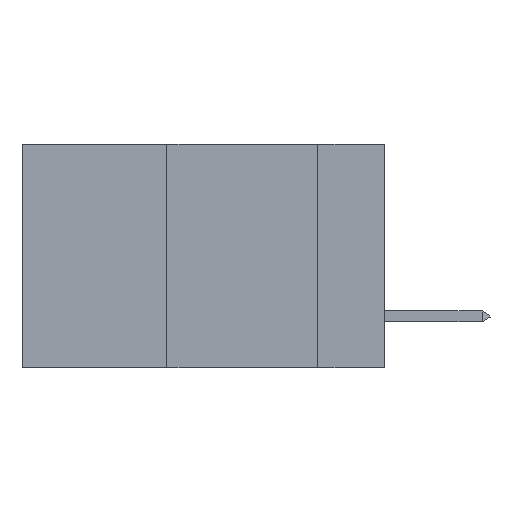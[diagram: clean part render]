
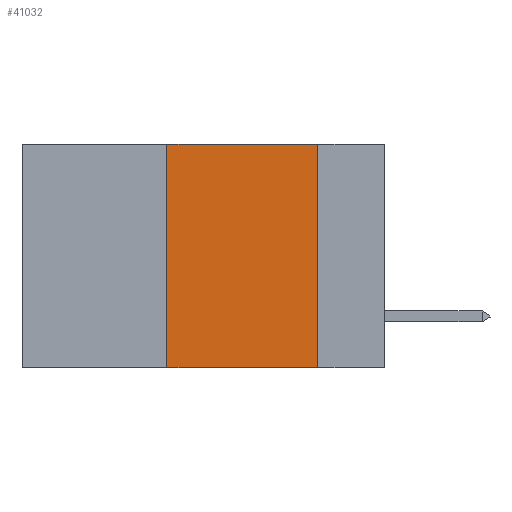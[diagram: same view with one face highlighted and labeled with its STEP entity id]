
A CAD part, left-side view. The second image highlights one B-rep face of the part: STEP entity #41032.
In plain terms, the highlighted planar face has unit normal (-1, 0, 0).
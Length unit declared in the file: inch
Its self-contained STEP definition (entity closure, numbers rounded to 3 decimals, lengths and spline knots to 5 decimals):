
#2736 = VERTEX_POINT ( 'NONE', #15024 ) ;
#3835 = CARTESIAN_POINT ( 'NONE',  ( 0., 0.11, 0. ) ) ;
#3850 = VECTOR ( 'NONE', #11219, 39.37008 ) ;
#7712 = EDGE_LOOP ( 'NONE', ( #29651, #24630, #30000, #11741 ) ) ;
#8691 = CARTESIAN_POINT ( 'NONE',  ( 0., 0.6, -0.37 ) ) ;
#10247 = CARTESIAN_POINT ( 'NONE',  ( 0., 0.36, -0.37 ) ) ;
#10599 = CARTESIAN_POINT ( 'NONE',  ( 0., 0.36, 0. ) ) ;
#11119 = CARTESIAN_POINT ( 'NONE',  ( 0., 0.36, 0. ) ) ;
#11219 = DIRECTION ( 'NONE',  ( 0., -1., 0. ) ) ;
#11250 = PLANE ( 'NONE',  #39860 ) ;
#11261 = LINE ( 'NONE', #27112, #23924 ) ;
#11718 = EDGE_CURVE ( 'NONE', #33342, #2736, #12462, .T. ) ;
#11741 = ORIENTED_EDGE ( 'NONE', *, *, #11718, .T. ) ;
#11813 = VECTOR ( 'NONE', #32857, 39.37008 ) ;
#12462 = LINE ( 'NONE', #8691, #3850 ) ;
#12538 = VECTOR ( 'NONE', #27082, 39.37008 ) ;
#13357 = DIRECTION ( 'NONE',  ( 1., 0., 0. ) ) ;
#15024 = CARTESIAN_POINT ( 'NONE',  ( 0., 0.11, -0.37 ) ) ;
#23924 = VECTOR ( 'NONE', #26682, 39.37008 ) ;
#24630 = ORIENTED_EDGE ( 'NONE', *, *, #35614, .F. ) ;
#26352 = EDGE_CURVE ( 'NONE', #33342, #26626, #29637, .T. ) ;
#26626 = VERTEX_POINT ( 'NONE', #10599 ) ;
#26682 = DIRECTION ( 'NONE',  ( 0., -1., 0. ) ) ;
#27082 = DIRECTION ( 'NONE',  ( 0., 0., 1. ) ) ;
#27112 = CARTESIAN_POINT ( 'NONE',  ( 0., 0.6, 0. ) ) ;
#29562 = DIRECTION ( 'NONE',  ( 0., 0., -1. ) ) ;
#29637 = LINE ( 'NONE', #11119, #12538 ) ;
#29651 = ORIENTED_EDGE ( 'NONE', *, *, #35589, .F. ) ;
#30000 = ORIENTED_EDGE ( 'NONE', *, *, #26352, .F. ) ;
#32002 = LINE ( 'NONE', #3835, #11813 ) ;
#32857 = DIRECTION ( 'NONE',  ( 0., 0., -1. ) ) ;
#33342 = VERTEX_POINT ( 'NONE', #10247 ) ;
#33530 = VERTEX_POINT ( 'NONE', #34791 ) ;
#33790 = CARTESIAN_POINT ( 'NONE',  ( 0., 0.6, 0. ) ) ;
#34791 = CARTESIAN_POINT ( 'NONE',  ( 0., 0.11, 0. ) ) ;
#35589 = EDGE_CURVE ( 'NONE', #33530, #2736, #32002, .T. ) ;
#35614 = EDGE_CURVE ( 'NONE', #26626, #33530, #11261, .T. ) ;
#39860 = AXIS2_PLACEMENT_3D ( 'NONE', #33790, #13357, #29562 ) ;
#40783 = FACE_OUTER_BOUND ( 'NONE', #7712, .T. ) ;
#41032 = ADVANCED_FACE ( 'NONE', ( #40783 ), #11250, .F. ) ;
